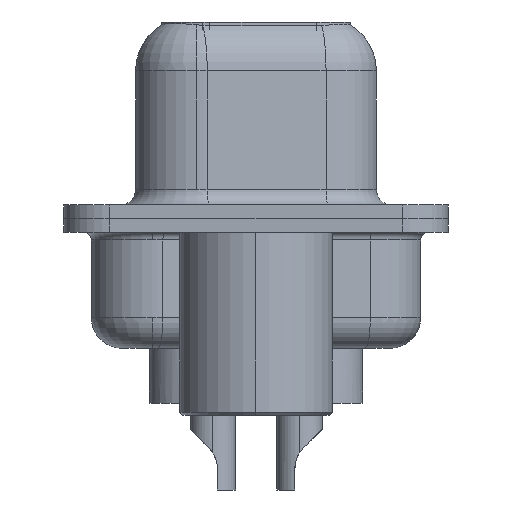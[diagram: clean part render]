
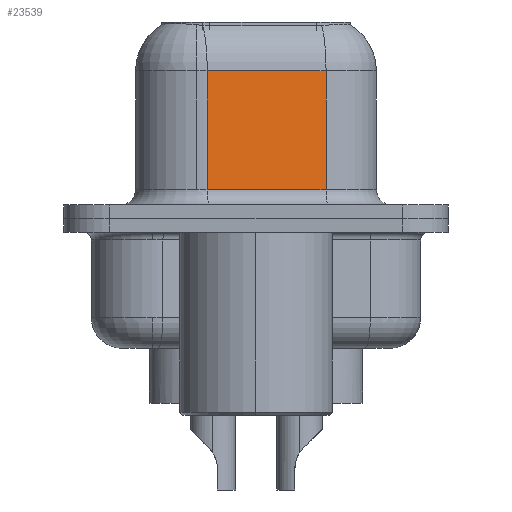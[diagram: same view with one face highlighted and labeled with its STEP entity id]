
A CAD part, left-side view. The second image highlights one B-rep face of the part: STEP entity #23539.
In plain terms, the highlighted planar face has unit normal (-0.985, -0.174, 0).
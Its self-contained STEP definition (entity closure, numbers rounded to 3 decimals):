
#642 = DIRECTION ( 'NONE',  ( -0.174, 0.985, 0. ) ) ;
#779 = LINE ( 'NONE', #12642, #12162 ) ;
#1680 = CARTESIAN_POINT ( 'NONE',  ( 5.038, -2.297, 0.95 ) ) ;
#2242 = AXIS2_PLACEMENT_3D ( 'NONE', #25388, #7317, #13387 ) ;
#3621 = VERTEX_POINT ( 'NONE', #17887 ) ;
#5020 = ORIENTED_EDGE ( 'NONE', *, *, #24752, .F. ) ;
#5470 = PLANE ( 'NONE',  #2242 ) ;
#6365 = CARTESIAN_POINT ( 'NONE',  ( 5.038, -2.297, 0.95 ) ) ;
#6562 = VERTEX_POINT ( 'NONE', #22754 ) ;
#6926 = EDGE_LOOP ( 'NONE', ( #5020, #19697, #8720, #15542 ) ) ;
#7317 = DIRECTION ( 'NONE',  ( 0.985, 0.174, 0. ) ) ;
#8396 = CARTESIAN_POINT ( 'NONE',  ( 4.35, 1.603, 0.95 ) ) ;
#8720 = ORIENTED_EDGE ( 'NONE', *, *, #21728, .T. ) ;
#9818 = EDGE_CURVE ( 'NONE', #9889, #11514, #11701, .T. ) ;
#9889 = VERTEX_POINT ( 'NONE', #8396 ) ;
#11514 = VERTEX_POINT ( 'NONE', #6365 ) ;
#11701 = LINE ( 'NONE', #1680, #11892 ) ;
#11892 = VECTOR ( 'NONE', #18552, 1000. ) ;
#12162 = VECTOR ( 'NONE', #642, 1000. ) ;
#12642 = CARTESIAN_POINT ( 'NONE',  ( 5.038, -2.297, 4.85 ) ) ;
#13387 = DIRECTION ( 'NONE',  ( -0.174, 0.985, 0. ) ) ;
#13784 = DIRECTION ( 'NONE',  ( 0., 0., -1. ) ) ;
#15313 = DIRECTION ( 'NONE',  ( 0., 0., -1. ) ) ;
#15542 = ORIENTED_EDGE ( 'NONE', *, *, #9818, .T. ) ;
#17191 = EDGE_CURVE ( 'NONE', #6562, #3621, #779, .T. ) ;
#17318 = LINE ( 'NONE', #25361, #17484 ) ;
#17347 = FACE_OUTER_BOUND ( 'NONE', #6926, .T. ) ;
#17484 = VECTOR ( 'NONE', #15313, 1000. ) ;
#17502 = CARTESIAN_POINT ( 'NONE',  ( 4.35, 1.603, 6.6 ) ) ;
#17887 = CARTESIAN_POINT ( 'NONE',  ( 4.35, 1.603, 4.85 ) ) ;
#18552 = DIRECTION ( 'NONE',  ( 0.174, -0.985, 0. ) ) ;
#19491 = LINE ( 'NONE', #17502, #24997 ) ;
#19697 = ORIENTED_EDGE ( 'NONE', *, *, #17191, .T. ) ;
#21728 = EDGE_CURVE ( 'NONE', #3621, #9889, #19491, .T. ) ;
#22754 = CARTESIAN_POINT ( 'NONE',  ( 5.038, -2.297, 4.85 ) ) ;
#23539 = ADVANCED_FACE ( 'NONE', ( #17347 ), #5470, .F. ) ;
#24752 = EDGE_CURVE ( 'NONE', #6562, #11514, #17318, .T. ) ;
#24997 = VECTOR ( 'NONE', #13784, 1000. ) ;
#25361 = CARTESIAN_POINT ( 'NONE',  ( 5.038, -2.297, 6.6 ) ) ;
#25388 = CARTESIAN_POINT ( 'NONE',  ( 5.038, -2.297, 6.6 ) ) ;
